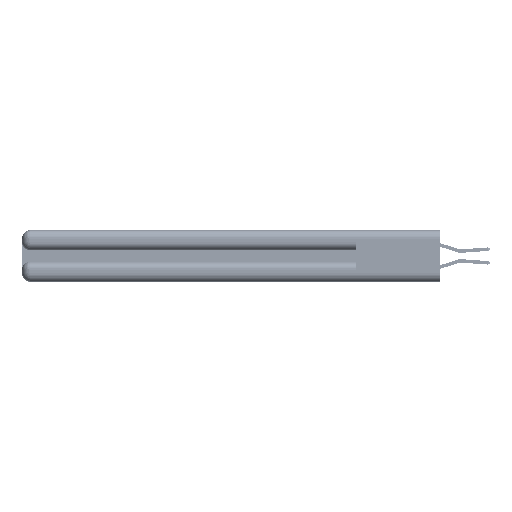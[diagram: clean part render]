
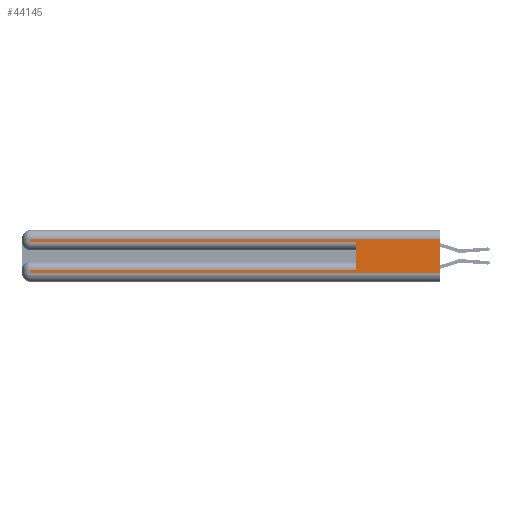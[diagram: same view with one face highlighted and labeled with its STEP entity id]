
A CAD part, left-side view. The second image highlights one B-rep face of the part: STEP entity #44145.
In plain terms, the highlighted planar face has unit normal (-1, 0, 0).
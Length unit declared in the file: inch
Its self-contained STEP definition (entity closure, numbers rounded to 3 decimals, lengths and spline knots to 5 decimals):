
#1056 = VECTOR ( 'NONE', #17314, 39.37008 ) ;
#1451 = CARTESIAN_POINT ( 'NONE',  ( 0., 0.6, 0.085 ) ) ;
#1457 = ORIENTED_EDGE ( 'NONE', *, *, #30002, .T. ) ;
#2413 = VECTOR ( 'NONE', #37296, 39.37008 ) ;
#2986 = LINE ( 'NONE', #8689, #23415 ) ;
#3011 = DIRECTION ( 'NONE',  ( 0., 0., -1. ) ) ;
#3104 = VECTOR ( 'NONE', #26728, 39.37008 ) ;
#3732 = CARTESIAN_POINT ( 'NONE',  ( 0., 2.94, 0.37 ) ) ;
#3740 = VERTEX_POINT ( 'NONE', #12445 ) ;
#4412 = CARTESIAN_POINT ( 'NONE',  ( 0., 2.94, 0.285 ) ) ;
#6726 = VERTEX_POINT ( 'NONE', #1451 ) ;
#7890 = PLANE ( 'NONE',  #28968 ) ;
#8689 = CARTESIAN_POINT ( 'NONE',  ( 0., 0.6, 0.145 ) ) ;
#9330 = FACE_OUTER_BOUND ( 'NONE', #32974, .T. ) ;
#10146 = VERTEX_POINT ( 'NONE', #4412 ) ;
#12203 = ORIENTED_EDGE ( 'NONE', *, *, #30519, .T. ) ;
#12445 = CARTESIAN_POINT ( 'NONE',  ( 0., 2.94, 0.31 ) ) ;
#12491 = ORIENTED_EDGE ( 'NONE', *, *, #35482, .T. ) ;
#12515 = VERTEX_POINT ( 'NONE', #47555 ) ;
#13032 = CARTESIAN_POINT ( 'NONE',  ( 0., 0., 0.31 ) ) ;
#13559 = LINE ( 'NONE', #45491, #35202 ) ;
#14194 = DIRECTION ( 'NONE',  ( 0., -1., 0. ) ) ;
#14447 = CARTESIAN_POINT ( 'NONE',  ( 0., 2.94, 0.06 ) ) ;
#14909 = LINE ( 'NONE', #34373, #46450 ) ;
#16664 = DIRECTION ( 'NONE',  ( 0., 0., 1. ) ) ;
#17262 = VERTEX_POINT ( 'NONE', #13032 ) ;
#17314 = DIRECTION ( 'NONE',  ( 0., -1., 0. ) ) ;
#18255 = CARTESIAN_POINT ( 'NONE',  ( 0., 0., 0.085 ) ) ;
#21935 = VECTOR ( 'NONE', #43379, 39.37008 ) ;
#22490 = VERTEX_POINT ( 'NONE', #23976 ) ;
#22815 = VECTOR ( 'NONE', #27979, 39.37008 ) ;
#23415 = VECTOR ( 'NONE', #16664, 39.37008 ) ;
#23976 = CARTESIAN_POINT ( 'NONE',  ( 0., 0., 0.06 ) ) ;
#24826 = DIRECTION ( 'NONE',  ( 0., 0., -1. ) ) ;
#25154 = ORIENTED_EDGE ( 'NONE', *, *, #44577, .F. ) ;
#26728 = DIRECTION ( 'NONE',  ( 0., 0., -1. ) ) ;
#27416 = CARTESIAN_POINT ( 'NONE',  ( 0., 0., 0.37 ) ) ;
#27602 = VERTEX_POINT ( 'NONE', #47978 ) ;
#27979 = DIRECTION ( 'NONE',  ( 0., 1., 0. ) ) ;
#28913 = CARTESIAN_POINT ( 'NONE',  ( 0., 0., 0.285 ) ) ;
#28968 = AXIS2_PLACEMENT_3D ( 'NONE', #40738, #48516, #24826 ) ;
#29383 = EDGE_CURVE ( 'NONE', #6726, #27602, #2986, .T. ) ;
#30002 = EDGE_CURVE ( 'NONE', #10146, #27602, #38274, .T. ) ;
#30519 = EDGE_CURVE ( 'NONE', #17262, #3740, #33964, .T. ) ;
#30697 = ORIENTED_EDGE ( 'NONE', *, *, #34873, .T. ) ;
#31090 = ORIENTED_EDGE ( 'NONE', *, *, #36074, .T. ) ;
#32877 = LINE ( 'NONE', #27416, #3104 ) ;
#32974 = EDGE_LOOP ( 'NONE', ( #25154, #12203, #34814, #1457, #38795, #12491, #30697, #31090 ) ) ;
#33964 = LINE ( 'NONE', #43867, #22815 ) ;
#34373 = CARTESIAN_POINT ( 'NONE',  ( 0., 2.94, 0.37 ) ) ;
#34814 = ORIENTED_EDGE ( 'NONE', *, *, #41150, .T. ) ;
#34873 = EDGE_CURVE ( 'NONE', #12515, #47674, #14909, .T. ) ;
#35202 = VECTOR ( 'NONE', #14194, 39.37008 ) ;
#35482 = EDGE_CURVE ( 'NONE', #6726, #12515, #45762, .T. ) ;
#36074 = EDGE_CURVE ( 'NONE', #47674, #22490, #13559, .T. ) ;
#37296 = DIRECTION ( 'NONE',  ( 0., 1., 0. ) ) ;
#38274 = LINE ( 'NONE', #28913, #1056 ) ;
#38795 = ORIENTED_EDGE ( 'NONE', *, *, #29383, .F. ) ;
#40738 = CARTESIAN_POINT ( 'NONE',  ( 0., 0., 0.37 ) ) ;
#41150 = EDGE_CURVE ( 'NONE', #3740, #10146, #44221, .T. ) ;
#43379 = DIRECTION ( 'NONE',  ( 0., 0., -1. ) ) ;
#43867 = CARTESIAN_POINT ( 'NONE',  ( 0., 0., 0.31 ) ) ;
#44145 = ADVANCED_FACE ( 'NONE', ( #9330 ), #7890, .F. ) ;
#44221 = LINE ( 'NONE', #3732, #21935 ) ;
#44577 = EDGE_CURVE ( 'NONE', #17262, #22490, #32877, .T. ) ;
#45491 = CARTESIAN_POINT ( 'NONE',  ( 0., 0., 0.06 ) ) ;
#45762 = LINE ( 'NONE', #18255, #2413 ) ;
#46450 = VECTOR ( 'NONE', #3011, 39.37008 ) ;
#47555 = CARTESIAN_POINT ( 'NONE',  ( 0., 2.94, 0.085 ) ) ;
#47674 = VERTEX_POINT ( 'NONE', #14447 ) ;
#47978 = CARTESIAN_POINT ( 'NONE',  ( 0., 0.6, 0.285 ) ) ;
#48516 = DIRECTION ( 'NONE',  ( 1., 0., 0. ) ) ;
